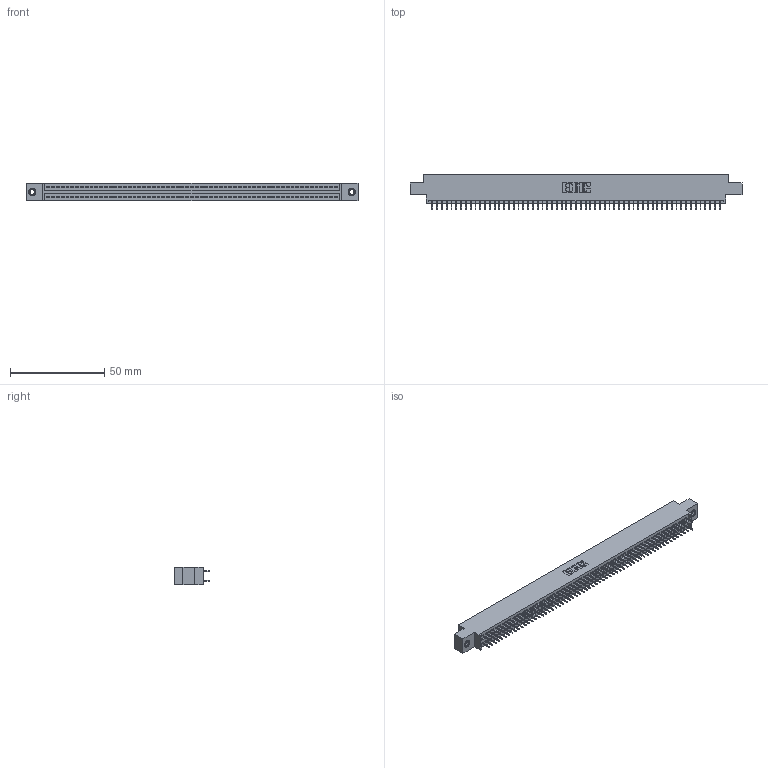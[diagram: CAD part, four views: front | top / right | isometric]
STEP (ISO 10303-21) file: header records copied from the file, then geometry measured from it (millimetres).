
FILE_DESCRIPTION (( 'STEP AP203' ), '1' );
FILE_NAME ('395-122-525-807.STEP', '2020-09-25T23:13:33', ( '' ), ( '' ), 'SwSTEP 2.0', 'SolidWorks 2020', '' );
FILE_SCHEMA (( 'CONFIG_CONTROL_DESIGN' ));
Length unit declared in the file: inch
Products named in the file (4): 345-292-001_345-293-125; 345-250-001_345-250-005-103; 345 Part_0.170 Offset - 0.156 Dia-TI; 395-122-525-807
Assembly tree (125 placements, depth 2):
  395-122-525-807
    345 Part_0.170 Offset - 0.156 Dia-TI
    345-292-001_345-293-125  x122
    345-250-001_345-250-005-103  x2
Bounding box: 176.15 x 18.72 x 9.4 mm (x, y, z)
Volume: 16959.9 mm3; surface area: 25003.9 mm2
Topology: 125 solids, 125 shells, 6778 faces, 19155 edges, 12274 vertices
Faces by surface type: plane 4874, cylinder 1888, cone 12, torus 4
Entity records: 46696 total; most frequent: CARTESIAN_POINT 7791, ORIENTED_EDGE 7718, DIRECTION 6873, EDGE_CURVE 3859, VECTOR 3467, LINE 3467, VERTEX_POINT 2564, AXIS2_PLACEMENT_3D 1703
